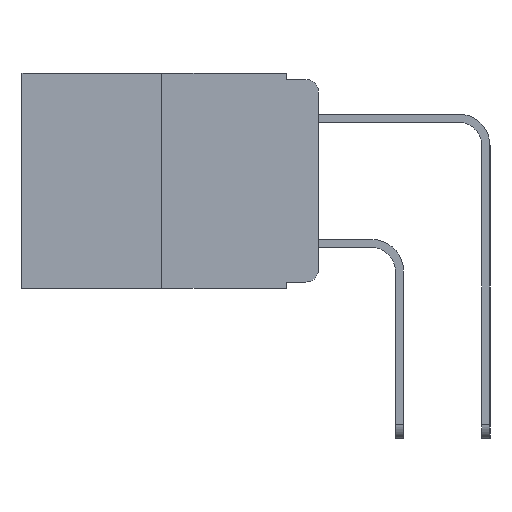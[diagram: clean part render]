
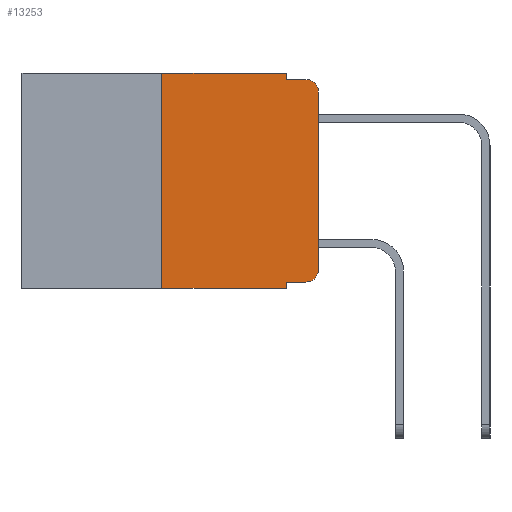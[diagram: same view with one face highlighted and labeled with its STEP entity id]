
A CAD part, left-side view. The second image highlights one B-rep face of the part: STEP entity #13253.
In plain terms, the highlighted planar face has unit normal (-1, 0, 0).
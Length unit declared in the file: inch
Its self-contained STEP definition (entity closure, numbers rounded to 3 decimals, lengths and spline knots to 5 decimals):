
#177 = ORIENTED_EDGE ( 'NONE', *, *, #6265, .T. ) ;
#276 = DIRECTION ( 'NONE',  ( 0., 0., -1. ) ) ;
#291 = VECTOR ( 'NONE', #11443, 39.37008 ) ;
#564 = VERTEX_POINT ( 'NONE', #18279 ) ;
#742 = DIRECTION ( 'NONE',  ( 0., 0., -1. ) ) ;
#902 = ORIENTED_EDGE ( 'NONE', *, *, #13378, .F. ) ;
#1020 = VERTEX_POINT ( 'NONE', #14267 ) ;
#1230 = DIRECTION ( 'NONE',  ( -1., 0., 0. ) ) ;
#1293 = VERTEX_POINT ( 'NONE', #13461 ) ;
#1340 = FACE_OUTER_BOUND ( 'NONE', #14913, .T. ) ;
#1429 = DIRECTION ( 'NONE',  ( 0., -1., 0. ) ) ;
#2114 = CARTESIAN_POINT ( 'NONE',  ( 0., 0.051, 0. ) ) ;
#2228 = CARTESIAN_POINT ( 'NONE',  ( 0., 0.473, 0. ) ) ;
#2486 = VECTOR ( 'NONE', #4793, 39.37008 ) ;
#2620 = CARTESIAN_POINT ( 'NONE',  ( 0., 0.02, -0.333 ) ) ;
#2933 = LINE ( 'NONE', #3296, #2486 ) ;
#2957 = VECTOR ( 'NONE', #15337, 39.37008 ) ;
#2999 = ORIENTED_EDGE ( 'NONE', *, *, #8700, .F. ) ;
#3296 = CARTESIAN_POINT ( 'NONE',  ( 0., 0.25, 0. ) ) ;
#3462 = ORIENTED_EDGE ( 'NONE', *, *, #9600, .F. ) ;
#3694 = ORIENTED_EDGE ( 'NONE', *, *, #15856, .F. ) ;
#3698 = VERTEX_POINT ( 'NONE', #2620 ) ;
#3718 = DIRECTION ( 'NONE',  ( 0., 0., -1. ) ) ;
#4793 = DIRECTION ( 'NONE',  ( 0., 0., 1. ) ) ;
#4862 = ORIENTED_EDGE ( 'NONE', *, *, #7350, .F. ) ;
#5121 = PLANE ( 'NONE',  #12075 ) ;
#5284 = AXIS2_PLACEMENT_3D ( 'NONE', #10025, #1230, #11455 ) ;
#5346 = CARTESIAN_POINT ( 'NONE',  ( 0., 0.051, -0.01 ) ) ;
#5890 = VECTOR ( 'NONE', #17819, 39.37008 ) ;
#6198 = ORIENTED_EDGE ( 'NONE', *, *, #10396, .T. ) ;
#6218 = ORIENTED_EDGE ( 'NONE', *, *, #16701, .T. ) ;
#6265 = EDGE_CURVE ( 'NONE', #15898, #1020, #13382, .T. ) ;
#6344 = LINE ( 'NONE', #10983, #5890 ) ;
#6951 = VECTOR ( 'NONE', #13762, 39.37008 ) ;
#6997 = LINE ( 'NONE', #10209, #14013 ) ;
#7038 = DIRECTION ( 'NONE',  ( 0., -1., 0. ) ) ;
#7350 = EDGE_CURVE ( 'NONE', #1293, #12878, #14394, .T. ) ;
#8180 = LINE ( 'NONE', #14658, #18371 ) ;
#8194 = VERTEX_POINT ( 'NONE', #9388 ) ;
#8446 = EDGE_CURVE ( 'NONE', #3698, #8194, #10229, .T. ) ;
#8700 = EDGE_CURVE ( 'NONE', #15898, #9678, #2933, .T. ) ;
#9163 = ORIENTED_EDGE ( 'NONE', *, *, #8446, .T. ) ;
#9182 = ORIENTED_EDGE ( 'NONE', *, *, #12144, .T. ) ;
#9388 = CARTESIAN_POINT ( 'NONE',  ( 0., 0., -0.313 ) ) ;
#9553 = DIRECTION ( 'NONE',  ( -1., 0., 0. ) ) ;
#9600 = EDGE_CURVE ( 'NONE', #9678, #17056, #6344, .T. ) ;
#9678 = VERTEX_POINT ( 'NONE', #15174 ) ;
#10025 = CARTESIAN_POINT ( 'NONE',  ( 0., 0.02, -0.313 ) ) ;
#10209 = CARTESIAN_POINT ( 'NONE',  ( 0., 0.051, -0.333 ) ) ;
#10229 = CIRCLE ( 'NONE', #5284, 0.02 ) ;
#10396 = EDGE_CURVE ( 'NONE', #564, #3698, #6997, .T. ) ;
#10622 = VECTOR ( 'NONE', #7038, 39.37008 ) ;
#10983 = CARTESIAN_POINT ( 'NONE',  ( 0., 0.473, 0. ) ) ;
#11443 = DIRECTION ( 'NONE',  ( 0., 0., 1. ) ) ;
#11455 = DIRECTION ( 'NONE',  ( 0., 0., -1. ) ) ;
#11529 = CARTESIAN_POINT ( 'NONE',  ( 0., 0., -0.03 ) ) ;
#11626 = AXIS2_PLACEMENT_3D ( 'NONE', #17774, #9553, #742 ) ;
#12075 = AXIS2_PLACEMENT_3D ( 'NONE', #2228, #12329, #3718 ) ;
#12144 = EDGE_CURVE ( 'NONE', #18061, #12878, #13957, .T. ) ;
#12329 = DIRECTION ( 'NONE',  ( 1., 0., 0. ) ) ;
#12878 = VERTEX_POINT ( 'NONE', #13935 ) ;
#13253 = ADVANCED_FACE ( 'NONE', ( #1340 ), #5121, .F. ) ;
#13378 = EDGE_CURVE ( 'NONE', #17056, #1293, #14331, .T. ) ;
#13382 = LINE ( 'NONE', #15390, #10622 ) ;
#13461 = CARTESIAN_POINT ( 'NONE',  ( 0., 0.051, -0.01 ) ) ;
#13762 = DIRECTION ( 'NONE',  ( 0., -1., 0. ) ) ;
#13935 = CARTESIAN_POINT ( 'NONE',  ( 0., 0.02, -0.01 ) ) ;
#13957 = CIRCLE ( 'NONE', #11626, 0.02 ) ;
#13974 = CARTESIAN_POINT ( 'NONE',  ( 0., 0.051, 0. ) ) ;
#14013 = VECTOR ( 'NONE', #1429, 39.37008 ) ;
#14267 = CARTESIAN_POINT ( 'NONE',  ( 0., 0.051, -0.343 ) ) ;
#14331 = LINE ( 'NONE', #13974, #2957 ) ;
#14394 = LINE ( 'NONE', #5346, #6951 ) ;
#14658 = CARTESIAN_POINT ( 'NONE',  ( 0., 0.051, 0. ) ) ;
#14913 = EDGE_LOOP ( 'NONE', ( #6218, #9182, #4862, #902, #3462, #2999, #177, #3694, #6198, #9163 ) ) ;
#15174 = CARTESIAN_POINT ( 'NONE',  ( 0., 0.25, 0. ) ) ;
#15337 = DIRECTION ( 'NONE',  ( 0., 0., -1. ) ) ;
#15390 = CARTESIAN_POINT ( 'NONE',  ( 0., 0.473, -0.343 ) ) ;
#15512 = LINE ( 'NONE', #18216, #291 ) ;
#15856 = EDGE_CURVE ( 'NONE', #564, #1020, #8180, .T. ) ;
#15898 = VERTEX_POINT ( 'NONE', #17468 ) ;
#16701 = EDGE_CURVE ( 'NONE', #8194, #18061, #15512, .T. ) ;
#17056 = VERTEX_POINT ( 'NONE', #2114 ) ;
#17468 = CARTESIAN_POINT ( 'NONE',  ( 0., 0.25, -0.343 ) ) ;
#17774 = CARTESIAN_POINT ( 'NONE',  ( 0., 0.02, -0.03 ) ) ;
#17819 = DIRECTION ( 'NONE',  ( 0., -1., 0. ) ) ;
#18061 = VERTEX_POINT ( 'NONE', #11529 ) ;
#18216 = CARTESIAN_POINT ( 'NONE',  ( 0., 0., 0. ) ) ;
#18279 = CARTESIAN_POINT ( 'NONE',  ( 0., 0.051, -0.333 ) ) ;
#18371 = VECTOR ( 'NONE', #276, 39.37008 ) ;
